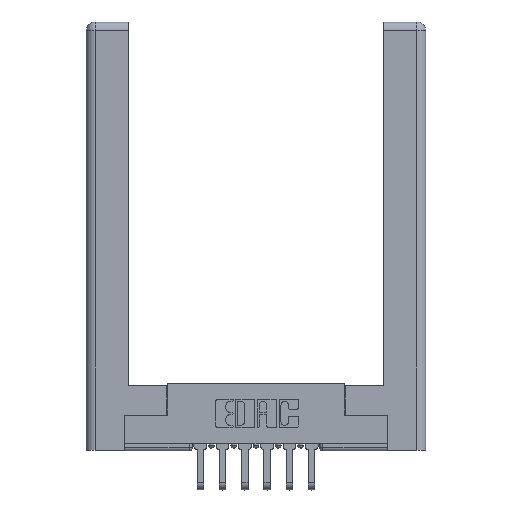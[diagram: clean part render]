
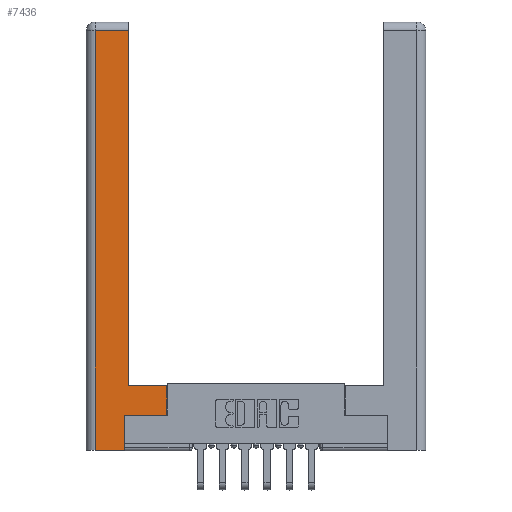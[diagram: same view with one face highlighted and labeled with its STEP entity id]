
A CAD part, top view. The second image highlights one B-rep face of the part: STEP entity #7436.
In plain terms, the highlighted planar face has unit normal (0, 0, 1).
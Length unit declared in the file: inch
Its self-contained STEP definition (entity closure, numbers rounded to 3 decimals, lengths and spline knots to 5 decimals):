
#427 = ORIENTED_EDGE ( 'NONE', *, *, #5441, .T. ) ;
#565 = VERTEX_POINT ( 'NONE', #11069 ) ;
#781 = VERTEX_POINT ( 'NONE', #13413 ) ;
#1024 = ORIENTED_EDGE ( 'NONE', *, *, #1548, .T. ) ;
#1422 = CARTESIAN_POINT ( 'NONE',  ( 0.295, 0.45, 0. ) ) ;
#1548 = EDGE_CURVE ( 'NONE', #8804, #12263, #12890, .T. ) ;
#1650 = LINE ( 'NONE', #12954, #5950 ) ;
#1716 = ORIENTED_EDGE ( 'NONE', *, *, #5323, .T. ) ;
#2563 = EDGE_CURVE ( 'NONE', #781, #6657, #12862, .T. ) ;
#2671 = CARTESIAN_POINT ( 'NONE',  ( 0.0615, 2.94, 0. ) ) ;
#3043 = LINE ( 'NONE', #10761, #5535 ) ;
#3467 = DIRECTION ( 'NONE',  ( 0., -1., 0. ) ) ;
#3515 = DIRECTION ( 'NONE',  ( 0., 1., 0. ) ) ;
#3613 = ORIENTED_EDGE ( 'NONE', *, *, #13827, .T. ) ;
#3631 = VECTOR ( 'NONE', #4870, 39.37008 ) ;
#4238 = ORIENTED_EDGE ( 'NONE', *, *, #2563, .T. ) ;
#4793 = VECTOR ( 'NONE', #3515, 39.37008 ) ;
#4870 = DIRECTION ( 'NONE',  ( -1., 0., 0. ) ) ;
#4886 = ORIENTED_EDGE ( 'NONE', *, *, #5317, .T. ) ;
#5317 = EDGE_CURVE ( 'NONE', #5541, #8804, #13642, .T. ) ;
#5323 = EDGE_CURVE ( 'NONE', #6657, #565, #13814, .T. ) ;
#5441 = EDGE_CURVE ( 'NONE', #12263, #7079, #10282, .T. ) ;
#5485 = VECTOR ( 'NONE', #9250, 39.37008 ) ;
#5535 = VECTOR ( 'NONE', #8447, 39.37008 ) ;
#5541 = VERTEX_POINT ( 'NONE', #7037 ) ;
#5702 = AXIS2_PLACEMENT_3D ( 'NONE', #13696, #9419, #13790 ) ;
#5950 = VECTOR ( 'NONE', #9841, 39.37008 ) ;
#6170 = PLANE ( 'NONE',  #5702 ) ;
#6244 = VECTOR ( 'NONE', #13309, 39.37008 ) ;
#6657 = VERTEX_POINT ( 'NONE', #7720 ) ;
#6717 = CARTESIAN_POINT ( 'NONE',  ( 0.0615, 0., 0. ) ) ;
#6831 = EDGE_CURVE ( 'NONE', #565, #7003, #3043, .T. ) ;
#6849 = FACE_OUTER_BOUND ( 'NONE', #8789, .T. ) ;
#7003 = VERTEX_POINT ( 'NONE', #7732 ) ;
#7037 = CARTESIAN_POINT ( 'NONE',  ( 0.265, 0.245, 0. ) ) ;
#7079 = VERTEX_POINT ( 'NONE', #1422 ) ;
#7436 = ADVANCED_FACE ( 'NONE', ( #6849 ), #6170, .F. ) ;
#7546 = CARTESIAN_POINT ( 'NONE',  ( 0.565, 0.245, 0. ) ) ;
#7720 = CARTESIAN_POINT ( 'NONE',  ( 0.0615, 2.94, 0. ) ) ;
#7732 = CARTESIAN_POINT ( 'NONE',  ( 0.265, 0., 0. ) ) ;
#8027 = CARTESIAN_POINT ( 'NONE',  ( 0.295, 0.45, 0. ) ) ;
#8302 = CARTESIAN_POINT ( 'NONE',  ( 0.565, 0.45, 0. ) ) ;
#8326 = LINE ( 'NONE', #13274, #4793 ) ;
#8361 = ORIENTED_EDGE ( 'NONE', *, *, #9398, .T. ) ;
#8447 = DIRECTION ( 'NONE',  ( 1., 0., 0. ) ) ;
#8789 = EDGE_LOOP ( 'NONE', ( #8361, #4238, #1716, #9343, #3613, #4886, #1024, #427 ) ) ;
#8804 = VERTEX_POINT ( 'NONE', #7546 ) ;
#9250 = DIRECTION ( 'NONE',  ( 0., 1., 0. ) ) ;
#9343 = ORIENTED_EDGE ( 'NONE', *, *, #6831, .T. ) ;
#9398 = EDGE_CURVE ( 'NONE', #7079, #781, #1650, .T. ) ;
#9419 = DIRECTION ( 'NONE',  ( 0., 0., -1. ) ) ;
#9790 = CARTESIAN_POINT ( 'NONE',  ( 0.565, 0.45, 0. ) ) ;
#9841 = DIRECTION ( 'NONE',  ( 0., 1., 0. ) ) ;
#10020 = DIRECTION ( 'NONE',  ( 1., 0., 0. ) ) ;
#10282 = LINE ( 'NONE', #8027, #6244 ) ;
#10761 = CARTESIAN_POINT ( 'NONE',  ( 0.265, 0., 0. ) ) ;
#10968 = VECTOR ( 'NONE', #3467, 39.37008 ) ;
#11069 = CARTESIAN_POINT ( 'NONE',  ( 0.0615, 0., 0. ) ) ;
#12263 = VERTEX_POINT ( 'NONE', #9790 ) ;
#12302 = VECTOR ( 'NONE', #10020, 39.37008 ) ;
#12862 = LINE ( 'NONE', #2671, #3631 ) ;
#12890 = LINE ( 'NONE', #8302, #5485 ) ;
#12954 = CARTESIAN_POINT ( 'NONE',  ( 0.295, 3., 0. ) ) ;
#13176 = CARTESIAN_POINT ( 'NONE',  ( 0.565, 0.245, 0. ) ) ;
#13274 = CARTESIAN_POINT ( 'NONE',  ( 0.265, 0.245, 0. ) ) ;
#13309 = DIRECTION ( 'NONE',  ( -1., 0., 0. ) ) ;
#13413 = CARTESIAN_POINT ( 'NONE',  ( 0.295, 2.94, 0. ) ) ;
#13642 = LINE ( 'NONE', #13176, #12302 ) ;
#13696 = CARTESIAN_POINT ( 'NONE',  ( 0., 0., 0. ) ) ;
#13790 = DIRECTION ( 'NONE',  ( -1., 0., 0. ) ) ;
#13814 = LINE ( 'NONE', #6717, #10968 ) ;
#13827 = EDGE_CURVE ( 'NONE', #7003, #5541, #8326, .T. ) ;
